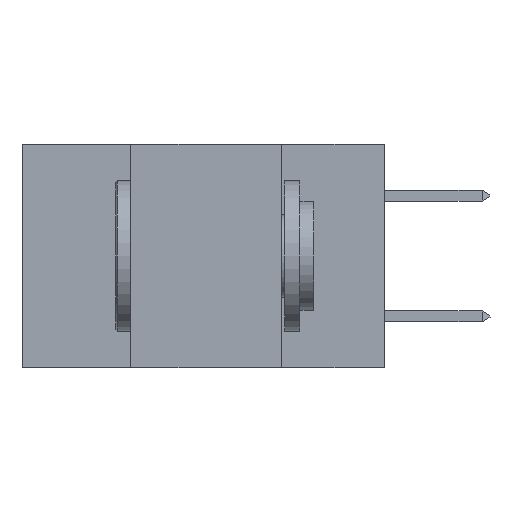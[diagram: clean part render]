
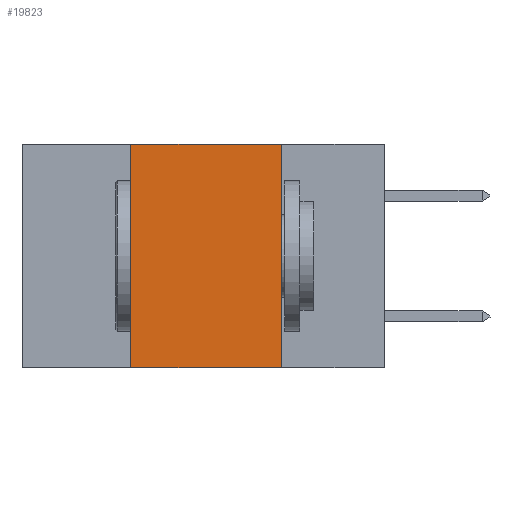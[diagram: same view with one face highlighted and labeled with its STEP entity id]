
A CAD part, left-side view. The second image highlights one B-rep face of the part: STEP entity #19823.
In plain terms, the highlighted planar face has unit normal (-1, 0, 0).
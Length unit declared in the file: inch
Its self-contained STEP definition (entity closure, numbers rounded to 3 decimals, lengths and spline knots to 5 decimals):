
#100 = VECTOR ( 'NONE', #9287, 39.37008 ) ;
#172 = ORIENTED_EDGE ( 'NONE', *, *, #10266, .F. ) ;
#518 = CARTESIAN_POINT ( 'NONE',  ( 0., 0.6, 0. ) ) ;
#1558 = PLANE ( 'NONE',  #17749 ) ;
#2629 = VECTOR ( 'NONE', #5714, 39.37008 ) ;
#3304 = CARTESIAN_POINT ( 'NONE',  ( 0., 0.6, 0. ) ) ;
#3743 = EDGE_CURVE ( 'NONE', #21635, #8835, #5414, .T. ) ;
#4748 = EDGE_CURVE ( 'NONE', #20488, #12537, #12996, .T. ) ;
#5075 = DIRECTION ( 'NONE',  ( 1., 0., 0. ) ) ;
#5086 = EDGE_CURVE ( 'NONE', #8835, #12537, #16299, .T. ) ;
#5413 = LINE ( 'NONE', #19913, #17933 ) ;
#5414 = LINE ( 'NONE', #518, #100 ) ;
#5714 = DIRECTION ( 'NONE',  ( 0., 0., -1. ) ) ;
#6668 = DIRECTION ( 'NONE',  ( 0., -1., 0. ) ) ;
#7480 = ORIENTED_EDGE ( 'NONE', *, *, #3743, .F. ) ;
#8835 = VERTEX_POINT ( 'NONE', #13264 ) ;
#8856 = EDGE_LOOP ( 'NONE', ( #15081, #7480, #172, #16272 ) ) ;
#9287 = DIRECTION ( 'NONE',  ( 0., -1., 0. ) ) ;
#10266 = EDGE_CURVE ( 'NONE', #20488, #21635, #5413, .T. ) ;
#10396 = CARTESIAN_POINT ( 'NONE',  ( 0., 0.42, -0.37 ) ) ;
#12537 = VERTEX_POINT ( 'NONE', #13115 ) ;
#12901 = CARTESIAN_POINT ( 'NONE',  ( 0., 0.17, 0. ) ) ;
#12996 = LINE ( 'NONE', #13932, #21640 ) ;
#13115 = CARTESIAN_POINT ( 'NONE',  ( 0., 0.17, -0.37 ) ) ;
#13264 = CARTESIAN_POINT ( 'NONE',  ( 0., 0.17, 0. ) ) ;
#13932 = CARTESIAN_POINT ( 'NONE',  ( 0., 0.6, -0.37 ) ) ;
#14669 = DIRECTION ( 'NONE',  ( 0., 0., 1. ) ) ;
#15081 = ORIENTED_EDGE ( 'NONE', *, *, #5086, .F. ) ;
#16272 = ORIENTED_EDGE ( 'NONE', *, *, #4748, .T. ) ;
#16299 = LINE ( 'NONE', #12901, #2629 ) ;
#17068 = FACE_OUTER_BOUND ( 'NONE', #8856, .T. ) ;
#17531 = DIRECTION ( 'NONE',  ( 0., 0., -1. ) ) ;
#17749 = AXIS2_PLACEMENT_3D ( 'NONE', #3304, #5075, #17531 ) ;
#17933 = VECTOR ( 'NONE', #14669, 39.37008 ) ;
#19823 = ADVANCED_FACE ( 'NONE', ( #17068 ), #1558, .F. ) ;
#19913 = CARTESIAN_POINT ( 'NONE',  ( 0., 0.42, 0. ) ) ;
#20144 = CARTESIAN_POINT ( 'NONE',  ( 0., 0.42, 0. ) ) ;
#20488 = VERTEX_POINT ( 'NONE', #10396 ) ;
#21635 = VERTEX_POINT ( 'NONE', #20144 ) ;
#21640 = VECTOR ( 'NONE', #6668, 39.37008 ) ;
